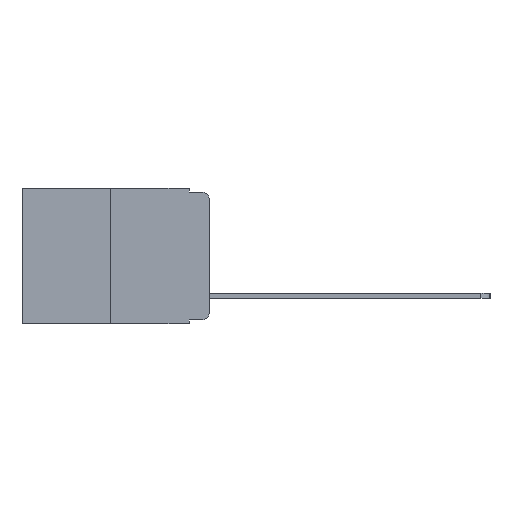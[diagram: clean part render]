
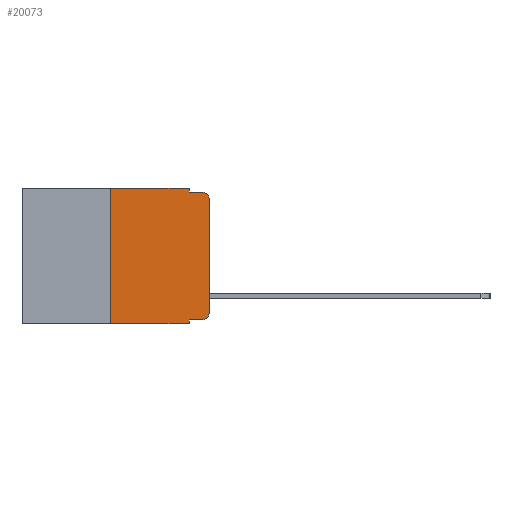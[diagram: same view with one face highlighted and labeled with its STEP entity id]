
A CAD part, left-side view. The second image highlights one B-rep face of the part: STEP entity #20073.
In plain terms, the highlighted planar face has unit normal (-1, 0, 0).
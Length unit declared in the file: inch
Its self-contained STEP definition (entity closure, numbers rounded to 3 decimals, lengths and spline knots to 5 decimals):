
#93 = VECTOR ( 'NONE', #18043, 39.37008 ) ;
#123 = CARTESIAN_POINT ( 'NONE',  ( 0., 0.051, -0.333 ) ) ;
#134 = VERTEX_POINT ( 'NONE', #123 ) ;
#138 = CARTESIAN_POINT ( 'NONE',  ( 0., 0.051, 0. ) ) ;
#304 = CARTESIAN_POINT ( 'NONE',  ( 0., 0.051, 0. ) ) ;
#584 = CARTESIAN_POINT ( 'NONE',  ( 0., 0.051, -0.343 ) ) ;
#683 = CARTESIAN_POINT ( 'NONE',  ( 0., 0., -0.313 ) ) ;
#796 = VECTOR ( 'NONE', #14755, 39.37008 ) ;
#892 = VERTEX_POINT ( 'NONE', #15754 ) ;
#1053 = CARTESIAN_POINT ( 'NONE',  ( 0., 0.02, -0.313 ) ) ;
#1214 = VERTEX_POINT ( 'NONE', #22937 ) ;
#1435 = LINE ( 'NONE', #3679, #16345 ) ;
#1500 = CARTESIAN_POINT ( 'NONE',  ( 0., 0.051, -0.01 ) ) ;
#1534 = CARTESIAN_POINT ( 'NONE',  ( 0., 0.02, -0.333 ) ) ;
#1656 = EDGE_CURVE ( 'NONE', #1214, #16886, #11765, .T. ) ;
#2432 = VERTEX_POINT ( 'NONE', #1534 ) ;
#2996 = DIRECTION ( 'NONE',  ( 0., 0., -1. ) ) ;
#3109 = CARTESIAN_POINT ( 'NONE',  ( 0., 0.473, -0.343 ) ) ;
#3490 = DIRECTION ( 'NONE',  ( -1., 0., 0. ) ) ;
#3569 = DIRECTION ( 'NONE',  ( 0., -1., 0. ) ) ;
#3579 = DIRECTION ( 'NONE',  ( 1., 0., 0. ) ) ;
#3679 = CARTESIAN_POINT ( 'NONE',  ( 0., 0.051, -0.333 ) ) ;
#4094 = ORIENTED_EDGE ( 'NONE', *, *, #4457, .F. ) ;
#4381 = CARTESIAN_POINT ( 'NONE',  ( 0., 0.473, 0. ) ) ;
#4457 = EDGE_CURVE ( 'NONE', #1214, #4995, #6128, .T. ) ;
#4995 = VERTEX_POINT ( 'NONE', #13285 ) ;
#5669 = DIRECTION ( 'NONE',  ( 0., -1., 0. ) ) ;
#5782 = EDGE_CURVE ( 'NONE', #7226, #14693, #18488, .T. ) ;
#6128 = LINE ( 'NONE', #7655, #15805 ) ;
#6855 = ORIENTED_EDGE ( 'NONE', *, *, #10963, .T. ) ;
#7084 = EDGE_CURVE ( 'NONE', #14693, #18930, #19026, .T. ) ;
#7226 = VERTEX_POINT ( 'NONE', #138 ) ;
#7446 = PLANE ( 'NONE',  #24749 ) ;
#7655 = CARTESIAN_POINT ( 'NONE',  ( 0., 0.25, 0. ) ) ;
#9284 = ORIENTED_EDGE ( 'NONE', *, *, #1656, .T. ) ;
#9678 = DIRECTION ( 'NONE',  ( 0., 0., -1. ) ) ;
#9935 = VECTOR ( 'NONE', #3569, 39.37008 ) ;
#10475 = LINE ( 'NONE', #4381, #93 ) ;
#10667 = EDGE_CURVE ( 'NONE', #4995, #7226, #10475, .T. ) ;
#10963 = EDGE_CURVE ( 'NONE', #892, #18930, #14080, .T. ) ;
#11385 = ORIENTED_EDGE ( 'NONE', *, *, #12254, .T. ) ;
#11765 = LINE ( 'NONE', #3109, #796 ) ;
#12254 = EDGE_CURVE ( 'NONE', #23904, #892, #24334, .T. ) ;
#12702 = VECTOR ( 'NONE', #15857, 39.37008 ) ;
#12711 = EDGE_LOOP ( 'NONE', ( #11385, #6855, #17147, #22313, #17767, #4094, #9284, #15021, #20210, #20803 ) ) ;
#13285 = CARTESIAN_POINT ( 'NONE',  ( 0., 0.25, 0. ) ) ;
#13472 = DIRECTION ( 'NONE',  ( 0., 0., 1. ) ) ;
#14013 = VECTOR ( 'NONE', #19506, 39.37008 ) ;
#14080 = CIRCLE ( 'NONE', #24118, 0.02 ) ;
#14660 = DIRECTION ( 'NONE',  ( -1., 0., 0. ) ) ;
#14693 = VERTEX_POINT ( 'NONE', #16737 ) ;
#14755 = DIRECTION ( 'NONE',  ( 0., -1., 0. ) ) ;
#15021 = ORIENTED_EDGE ( 'NONE', *, *, #23139, .F. ) ;
#15127 = CARTESIAN_POINT ( 'NONE',  ( 0., 0.02, -0.03 ) ) ;
#15205 = CARTESIAN_POINT ( 'NONE',  ( 0., 0.473, 0. ) ) ;
#15431 = CARTESIAN_POINT ( 'NONE',  ( 0., 0.02, -0.01 ) ) ;
#15754 = CARTESIAN_POINT ( 'NONE',  ( 0., 0., -0.03 ) ) ;
#15805 = VECTOR ( 'NONE', #13472, 39.37008 ) ;
#15857 = DIRECTION ( 'NONE',  ( 0., 0., -1. ) ) ;
#16345 = VECTOR ( 'NONE', #5669, 39.37008 ) ;
#16737 = CARTESIAN_POINT ( 'NONE',  ( 0., 0.051, -0.01 ) ) ;
#16886 = VERTEX_POINT ( 'NONE', #584 ) ;
#17084 = DIRECTION ( 'NONE',  ( 0., 0., -1. ) ) ;
#17147 = ORIENTED_EDGE ( 'NONE', *, *, #7084, .F. ) ;
#17169 = DIRECTION ( 'NONE',  ( 0., 0., -1. ) ) ;
#17548 = CARTESIAN_POINT ( 'NONE',  ( 0., 0., 0. ) ) ;
#17767 = ORIENTED_EDGE ( 'NONE', *, *, #10667, .F. ) ;
#18043 = DIRECTION ( 'NONE',  ( 0., -1., 0. ) ) ;
#18488 = LINE ( 'NONE', #304, #12702 ) ;
#18930 = VERTEX_POINT ( 'NONE', #15431 ) ;
#19026 = LINE ( 'NONE', #1500, #9935 ) ;
#19252 = EDGE_CURVE ( 'NONE', #2432, #23904, #19507, .T. ) ;
#19328 = CARTESIAN_POINT ( 'NONE',  ( 0., 0.051, 0. ) ) ;
#19506 = DIRECTION ( 'NONE',  ( 0., 0., 1. ) ) ;
#19507 = CIRCLE ( 'NONE', #22310, 0.02 ) ;
#20073 = ADVANCED_FACE ( 'NONE', ( #21877 ), #7446, .F. ) ;
#20210 = ORIENTED_EDGE ( 'NONE', *, *, #21846, .T. ) ;
#20803 = ORIENTED_EDGE ( 'NONE', *, *, #19252, .T. ) ;
#21645 = VECTOR ( 'NONE', #9678, 39.37008 ) ;
#21846 = EDGE_CURVE ( 'NONE', #134, #2432, #1435, .T. ) ;
#21877 = FACE_OUTER_BOUND ( 'NONE', #12711, .T. ) ;
#22257 = LINE ( 'NONE', #19328, #21645 ) ;
#22310 = AXIS2_PLACEMENT_3D ( 'NONE', #1053, #14660, #2996 ) ;
#22313 = ORIENTED_EDGE ( 'NONE', *, *, #5782, .F. ) ;
#22937 = CARTESIAN_POINT ( 'NONE',  ( 0., 0.25, -0.343 ) ) ;
#23139 = EDGE_CURVE ( 'NONE', #134, #16886, #22257, .T. ) ;
#23904 = VERTEX_POINT ( 'NONE', #683 ) ;
#24118 = AXIS2_PLACEMENT_3D ( 'NONE', #15127, #3490, #17084 ) ;
#24334 = LINE ( 'NONE', #17548, #14013 ) ;
#24749 = AXIS2_PLACEMENT_3D ( 'NONE', #15205, #3579, #17169 ) ;
